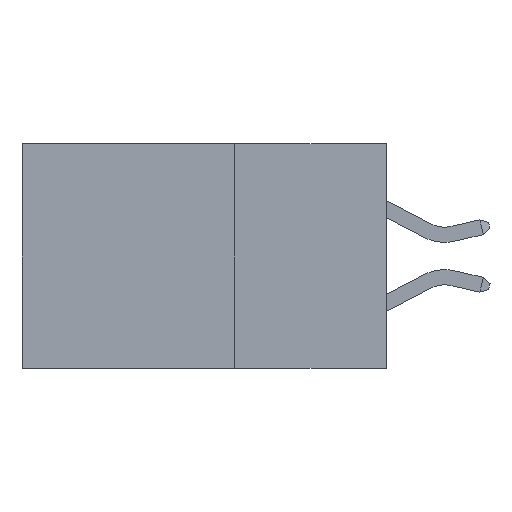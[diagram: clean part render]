
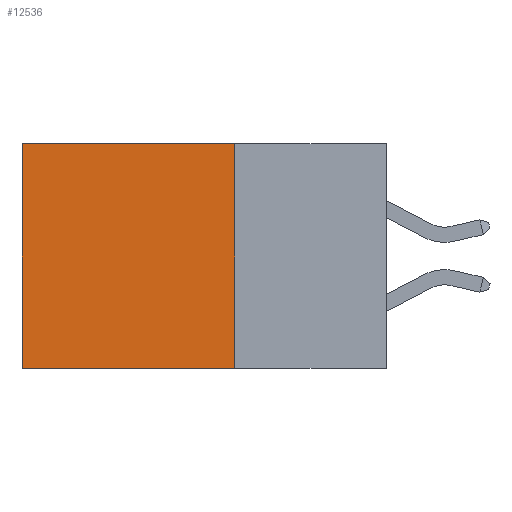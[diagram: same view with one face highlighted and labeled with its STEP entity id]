
A CAD part, left-side view. The second image highlights one B-rep face of the part: STEP entity #12536.
In plain terms, the highlighted planar face has unit normal (-1, 0, 0).
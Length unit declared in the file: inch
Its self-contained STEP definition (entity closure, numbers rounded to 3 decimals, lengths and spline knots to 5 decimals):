
#92 = CARTESIAN_POINT ( 'NONE',  ( 0.2615, 0.25, 0. ) ) ;
#630 = VERTEX_POINT ( 'NONE', #10885 ) ;
#952 = ORIENTED_EDGE ( 'NONE', *, *, #18010, .F. ) ;
#1012 = LINE ( 'NONE', #7151, #15813 ) ;
#1241 = DIRECTION ( 'NONE',  ( 0., 1., 0. ) ) ;
#1543 = ORIENTED_EDGE ( 'NONE', *, *, #16890, .F. ) ;
#2569 = DIRECTION ( 'NONE',  ( 0., 0., -1. ) ) ;
#2714 = LINE ( 'NONE', #92, #9936 ) ;
#3236 = ORIENTED_EDGE ( 'NONE', *, *, #9576, .T. ) ;
#3787 = CARTESIAN_POINT ( 'NONE',  ( 0.2615, 0.25, -0.37 ) ) ;
#4250 = LINE ( 'NONE', #3787, #11357 ) ;
#6246 = VECTOR ( 'NONE', #2569, 39.37008 ) ;
#6675 = PLANE ( 'NONE',  #17288 ) ;
#6846 = CARTESIAN_POINT ( 'NONE',  ( 0.2615, 0.6, 0. ) ) ;
#7015 = CARTESIAN_POINT ( 'NONE',  ( 0.2615, 0.6, -0.37 ) ) ;
#7151 = CARTESIAN_POINT ( 'NONE',  ( 0.2615, 0.25, -0.37 ) ) ;
#8107 = DIRECTION ( 'NONE',  ( 1., 0., 0. ) ) ;
#8128 = CARTESIAN_POINT ( 'NONE',  ( 0.2615, 0.6, -0.37 ) ) ;
#8332 = VERTEX_POINT ( 'NONE', #8128 ) ;
#8731 = VERTEX_POINT ( 'NONE', #16572 ) ;
#9154 = ORIENTED_EDGE ( 'NONE', *, *, #13944, .T. ) ;
#9197 = FACE_OUTER_BOUND ( 'NONE', #16056, .T. ) ;
#9576 = EDGE_CURVE ( 'NONE', #630, #10487, #2714, .T. ) ;
#9936 = VECTOR ( 'NONE', #14596, 39.37008 ) ;
#10487 = VERTEX_POINT ( 'NONE', #6846 ) ;
#10885 = CARTESIAN_POINT ( 'NONE',  ( 0.2615, 0.25, 0. ) ) ;
#11357 = VECTOR ( 'NONE', #16507, 39.37008 ) ;
#12536 = ADVANCED_FACE ( 'NONE', ( #9197 ), #6675, .F. ) ;
#13252 = LINE ( 'NONE', #7015, #6246 ) ;
#13944 = EDGE_CURVE ( 'NONE', #10487, #8332, #13252, .T. ) ;
#14596 = DIRECTION ( 'NONE',  ( 0., 1., 0. ) ) ;
#15813 = VECTOR ( 'NONE', #1241, 39.37008 ) ;
#16056 = EDGE_LOOP ( 'NONE', ( #9154, #1543, #952, #3236 ) ) ;
#16433 = CARTESIAN_POINT ( 'NONE',  ( 0.2615, 0.25, -0.37 ) ) ;
#16507 = DIRECTION ( 'NONE',  ( 0., 0., -1. ) ) ;
#16572 = CARTESIAN_POINT ( 'NONE',  ( 0.2615, 0.25, -0.37 ) ) ;
#16890 = EDGE_CURVE ( 'NONE', #8731, #8332, #1012, .T. ) ;
#17288 = AXIS2_PLACEMENT_3D ( 'NONE', #16433, #8107, #17827 ) ;
#17827 = DIRECTION ( 'NONE',  ( 0., 0., -1. ) ) ;
#18010 = EDGE_CURVE ( 'NONE', #630, #8731, #4250, .T. ) ;
